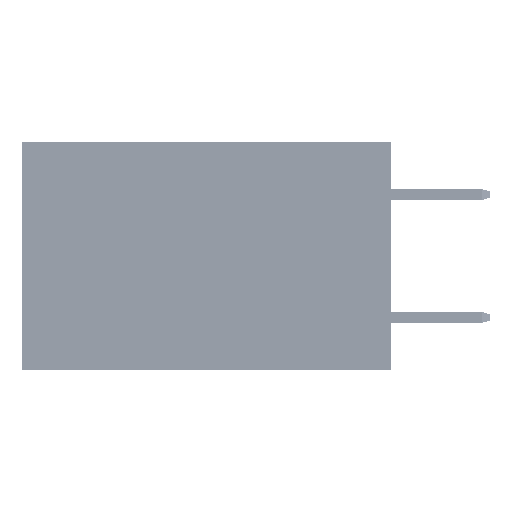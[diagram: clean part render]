
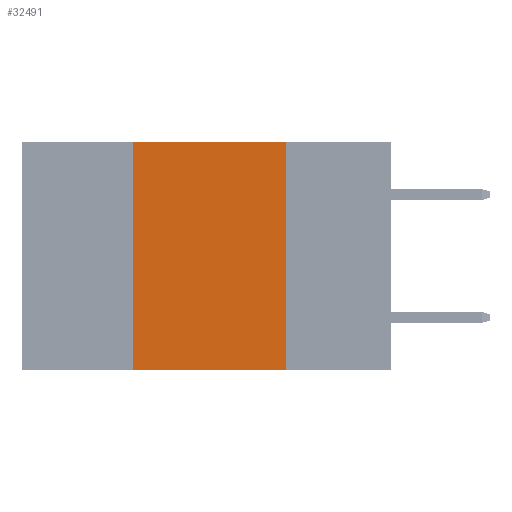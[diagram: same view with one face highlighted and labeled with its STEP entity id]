
A CAD part, left-side view. The second image highlights one B-rep face of the part: STEP entity #32491.
In plain terms, the highlighted planar face has unit normal (-1, 0, 0).
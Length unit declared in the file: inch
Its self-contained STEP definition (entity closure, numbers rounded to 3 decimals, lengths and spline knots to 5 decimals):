
#1296 = CARTESIAN_POINT ( 'NONE',  ( 0., 0.17, -0.37 ) ) ;
#2160 = ORIENTED_EDGE ( 'NONE', *, *, #9015, .T. ) ;
#2820 = ORIENTED_EDGE ( 'NONE', *, *, #16444, .F. ) ;
#3847 = VECTOR ( 'NONE', #35367, 39.37008 ) ;
#4079 = ORIENTED_EDGE ( 'NONE', *, *, #20457, .F. ) ;
#6175 = VERTEX_POINT ( 'NONE', #1296 ) ;
#7660 = VECTOR ( 'NONE', #28450, 39.37008 ) ;
#8195 = DIRECTION ( 'NONE',  ( 0., -1., 0. ) ) ;
#9015 = EDGE_CURVE ( 'NONE', #35064, #6175, #21905, .T. ) ;
#9675 = VECTOR ( 'NONE', #8195, 39.37008 ) ;
#12014 = LINE ( 'NONE', #30304, #9675 ) ;
#12395 = EDGE_CURVE ( 'NONE', #14069, #29962, #12014, .T. ) ;
#14069 = VERTEX_POINT ( 'NONE', #33041 ) ;
#15126 = CARTESIAN_POINT ( 'NONE',  ( 0., 0.42, -0.37 ) ) ;
#16363 = LINE ( 'NONE', #24736, #7660 ) ;
#16444 = EDGE_CURVE ( 'NONE', #35064, #14069, #16363, .T. ) ;
#16501 = CARTESIAN_POINT ( 'NONE',  ( 0., 0.17, 0. ) ) ;
#19889 = DIRECTION ( 'NONE',  ( 0., -1., 0. ) ) ;
#20457 = EDGE_CURVE ( 'NONE', #29962, #6175, #41639, .T. ) ;
#21905 = LINE ( 'NONE', #27532, #42827 ) ;
#22073 = CARTESIAN_POINT ( 'NONE',  ( 0., 0.6, 0. ) ) ;
#22244 = DIRECTION ( 'NONE',  ( 1., 0., 0. ) ) ;
#22246 = CARTESIAN_POINT ( 'NONE',  ( 0., 0.17, 0. ) ) ;
#22554 = DIRECTION ( 'NONE',  ( 0., 0., -1. ) ) ;
#24736 = CARTESIAN_POINT ( 'NONE',  ( 0., 0.42, 0. ) ) ;
#27532 = CARTESIAN_POINT ( 'NONE',  ( 0., 0.6, -0.37 ) ) ;
#27537 = AXIS2_PLACEMENT_3D ( 'NONE', #22073, #22244, #22554 ) ;
#28450 = DIRECTION ( 'NONE',  ( 0., 0., 1. ) ) ;
#29399 = PLANE ( 'NONE',  #27537 ) ;
#29962 = VERTEX_POINT ( 'NONE', #22246 ) ;
#30304 = CARTESIAN_POINT ( 'NONE',  ( 0., 0.6, 0. ) ) ;
#32491 = ADVANCED_FACE ( 'NONE', ( #43755 ), #29399, .F. ) ;
#33041 = CARTESIAN_POINT ( 'NONE',  ( 0., 0.42, 0. ) ) ;
#35064 = VERTEX_POINT ( 'NONE', #15126 ) ;
#35367 = DIRECTION ( 'NONE',  ( 0., 0., -1. ) ) ;
#36385 = ORIENTED_EDGE ( 'NONE', *, *, #12395, .F. ) ;
#41639 = LINE ( 'NONE', #16501, #3847 ) ;
#42326 = EDGE_LOOP ( 'NONE', ( #4079, #36385, #2820, #2160 ) ) ;
#42827 = VECTOR ( 'NONE', #19889, 39.37008 ) ;
#43755 = FACE_OUTER_BOUND ( 'NONE', #42326, .T. ) ;
